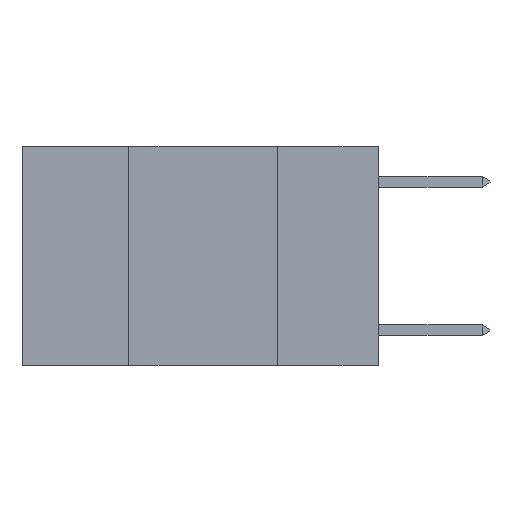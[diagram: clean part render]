
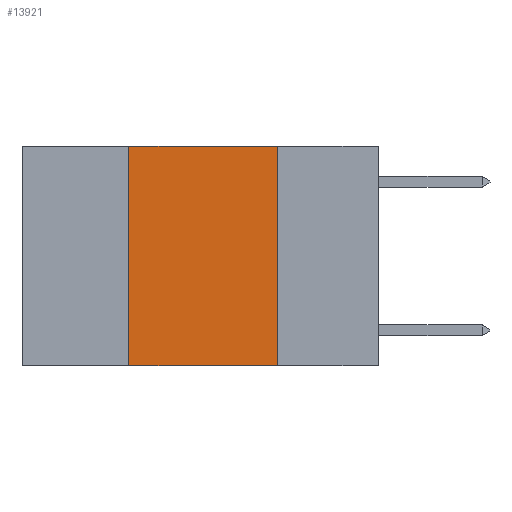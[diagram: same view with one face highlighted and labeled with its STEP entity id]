
A CAD part, left-side view. The second image highlights one B-rep face of the part: STEP entity #13921.
In plain terms, the highlighted planar face has unit normal (-1, 0, 0).
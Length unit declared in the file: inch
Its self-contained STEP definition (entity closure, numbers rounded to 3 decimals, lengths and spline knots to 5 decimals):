
#843 = CARTESIAN_POINT ( 'NONE',  ( 0., 0.42, -0.37 ) ) ;
#987 = DIRECTION ( 'NONE',  ( 0., 0., -1. ) ) ;
#1382 = CARTESIAN_POINT ( 'NONE',  ( 0., 0.6, -0.37 ) ) ;
#1635 = VERTEX_POINT ( 'NONE', #9248 ) ;
#1825 = LINE ( 'NONE', #13189, #4641 ) ;
#2352 = DIRECTION ( 'NONE',  ( 0., 0., 1. ) ) ;
#2735 = LINE ( 'NONE', #1382, #4414 ) ;
#3554 = CARTESIAN_POINT ( 'NONE',  ( 0., 0.42, 0. ) ) ;
#3712 = VERTEX_POINT ( 'NONE', #8252 ) ;
#3839 = EDGE_LOOP ( 'NONE', ( #11140, #14302, #15396, #15137 ) ) ;
#4414 = VECTOR ( 'NONE', #8541, 39.37008 ) ;
#4563 = PLANE ( 'NONE',  #13194 ) ;
#4641 = VECTOR ( 'NONE', #8568, 39.37008 ) ;
#5829 = VECTOR ( 'NONE', #12760, 39.37008 ) ;
#6360 = VECTOR ( 'NONE', #2352, 39.37008 ) ;
#6745 = LINE ( 'NONE', #3554, #6360 ) ;
#6953 = EDGE_CURVE ( 'NONE', #11422, #1635, #6745, .T. ) ;
#7698 = EDGE_CURVE ( 'NONE', #3712, #8717, #1825, .T. ) ;
#8151 = DIRECTION ( 'NONE',  ( 1., 0., 0. ) ) ;
#8252 = CARTESIAN_POINT ( 'NONE',  ( 0., 0.17, 0. ) ) ;
#8428 = FACE_OUTER_BOUND ( 'NONE', #3839, .T. ) ;
#8541 = DIRECTION ( 'NONE',  ( 0., -1., 0. ) ) ;
#8568 = DIRECTION ( 'NONE',  ( 0., 0., -1. ) ) ;
#8717 = VERTEX_POINT ( 'NONE', #9387 ) ;
#8914 = EDGE_CURVE ( 'NONE', #11422, #8717, #2735, .T. ) ;
#9248 = CARTESIAN_POINT ( 'NONE',  ( 0., 0.42, 0. ) ) ;
#9387 = CARTESIAN_POINT ( 'NONE',  ( 0., 0.17, -0.37 ) ) ;
#11140 = ORIENTED_EDGE ( 'NONE', *, *, #7698, .F. ) ;
#11422 = VERTEX_POINT ( 'NONE', #843 ) ;
#12760 = DIRECTION ( 'NONE',  ( 0., -1., 0. ) ) ;
#12824 = CARTESIAN_POINT ( 'NONE',  ( 0., 0.6, 0. ) ) ;
#13189 = CARTESIAN_POINT ( 'NONE',  ( 0., 0.17, 0. ) ) ;
#13194 = AXIS2_PLACEMENT_3D ( 'NONE', #12824, #8151, #987 ) ;
#13921 = ADVANCED_FACE ( 'NONE', ( #8428 ), #4563, .F. ) ;
#14302 = ORIENTED_EDGE ( 'NONE', *, *, #14540, .F. ) ;
#14540 = EDGE_CURVE ( 'NONE', #1635, #3712, #15227, .T. ) ;
#15134 = CARTESIAN_POINT ( 'NONE',  ( 0., 0.6, 0. ) ) ;
#15137 = ORIENTED_EDGE ( 'NONE', *, *, #8914, .T. ) ;
#15227 = LINE ( 'NONE', #15134, #5829 ) ;
#15396 = ORIENTED_EDGE ( 'NONE', *, *, #6953, .F. ) ;
